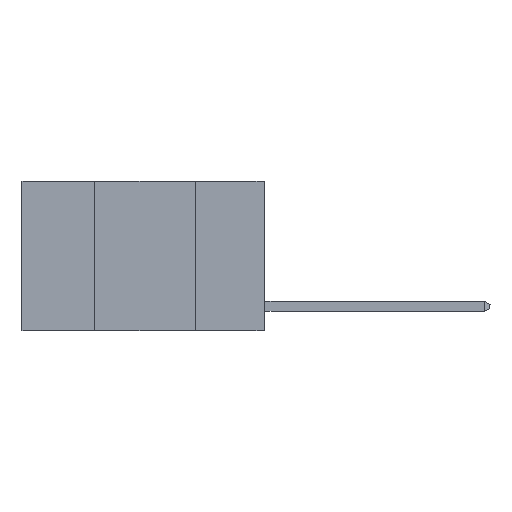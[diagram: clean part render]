
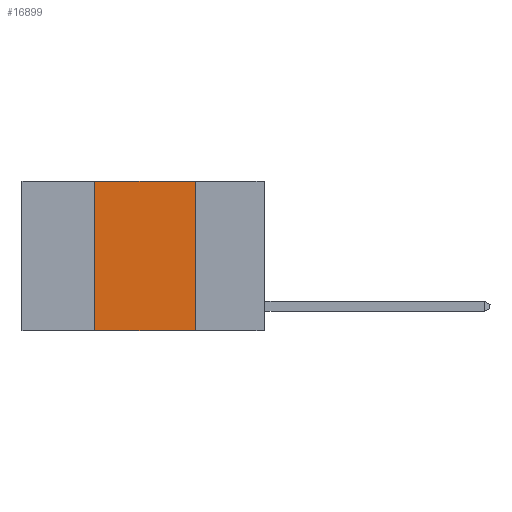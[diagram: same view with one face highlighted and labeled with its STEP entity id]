
A CAD part, left-side view. The second image highlights one B-rep face of the part: STEP entity #16899.
In plain terms, the highlighted planar face has unit normal (-1, 0, 0).
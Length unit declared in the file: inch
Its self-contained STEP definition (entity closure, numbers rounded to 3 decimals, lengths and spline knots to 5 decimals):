
#152 = DIRECTION ( 'NONE',  ( 0., -1., 0. ) ) ;
#344 = DIRECTION ( 'NONE',  ( 0., 0., 1. ) ) ;
#1428 = ORIENTED_EDGE ( 'NONE', *, *, #13079, .F. ) ;
#1662 = EDGE_LOOP ( 'NONE', ( #6790, #12787, #1428, #20100 ) ) ;
#1804 = VERTEX_POINT ( 'NONE', #28580 ) ;
#3163 = PLANE ( 'NONE',  #25918 ) ;
#4541 = EDGE_CURVE ( 'NONE', #1804, #26669, #22403, .T. ) ;
#5168 = VERTEX_POINT ( 'NONE', #11116 ) ;
#6095 = DIRECTION ( 'NONE',  ( 0., 0., -1. ) ) ;
#6790 = ORIENTED_EDGE ( 'NONE', *, *, #22963, .F. ) ;
#6867 = LINE ( 'NONE', #16187, #23321 ) ;
#7831 = LINE ( 'NONE', #27142, #24970 ) ;
#10036 = DIRECTION ( 'NONE',  ( 0., 0., -1. ) ) ;
#11116 = CARTESIAN_POINT ( 'NONE',  ( 0., 0.42, -0.37 ) ) ;
#11147 = CARTESIAN_POINT ( 'NONE',  ( 0., 0.6, 0. ) ) ;
#11852 = LINE ( 'NONE', #26247, #28901 ) ;
#12787 = ORIENTED_EDGE ( 'NONE', *, *, #4541, .F. ) ;
#13079 = EDGE_CURVE ( 'NONE', #5168, #1804, #6867, .T. ) ;
#16187 = CARTESIAN_POINT ( 'NONE',  ( 0., 0.42, 0. ) ) ;
#16558 = CARTESIAN_POINT ( 'NONE',  ( 0., 0.6, 0. ) ) ;
#16899 = ADVANCED_FACE ( 'NONE', ( #23670 ), #3163, .F. ) ;
#17398 = CARTESIAN_POINT ( 'NONE',  ( 0., 0.17, 0. ) ) ;
#17852 = DIRECTION ( 'NONE',  ( 0., -1., 0. ) ) ;
#20100 = ORIENTED_EDGE ( 'NONE', *, *, #25026, .T. ) ;
#22403 = LINE ( 'NONE', #11147, #27655 ) ;
#22445 = CARTESIAN_POINT ( 'NONE',  ( 0., 0.17, -0.37 ) ) ;
#22963 = EDGE_CURVE ( 'NONE', #26669, #26853, #11852, .T. ) ;
#23321 = VECTOR ( 'NONE', #344, 39.37008 ) ;
#23382 = DIRECTION ( 'NONE',  ( 1., 0., 0. ) ) ;
#23670 = FACE_OUTER_BOUND ( 'NONE', #1662, .T. ) ;
#24970 = VECTOR ( 'NONE', #152, 39.37008 ) ;
#25026 = EDGE_CURVE ( 'NONE', #5168, #26853, #7831, .T. ) ;
#25918 = AXIS2_PLACEMENT_3D ( 'NONE', #16558, #23382, #10036 ) ;
#26247 = CARTESIAN_POINT ( 'NONE',  ( 0., 0.17, 0. ) ) ;
#26669 = VERTEX_POINT ( 'NONE', #17398 ) ;
#26853 = VERTEX_POINT ( 'NONE', #22445 ) ;
#27142 = CARTESIAN_POINT ( 'NONE',  ( 0., 0.6, -0.37 ) ) ;
#27655 = VECTOR ( 'NONE', #17852, 39.37008 ) ;
#28580 = CARTESIAN_POINT ( 'NONE',  ( 0., 0.42, 0. ) ) ;
#28901 = VECTOR ( 'NONE', #6095, 39.37008 ) ;
